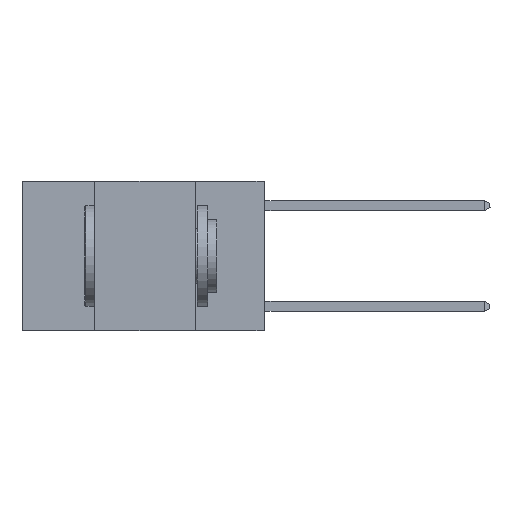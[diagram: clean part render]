
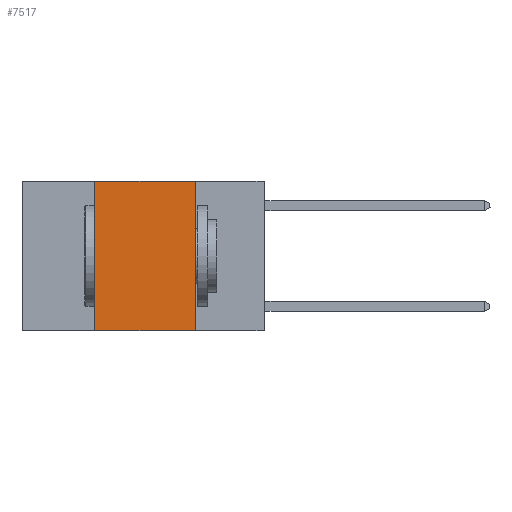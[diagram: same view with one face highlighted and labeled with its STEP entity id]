
A CAD part, left-side view. The second image highlights one B-rep face of the part: STEP entity #7517.
In plain terms, the highlighted planar face has unit normal (-1, 0, 0).
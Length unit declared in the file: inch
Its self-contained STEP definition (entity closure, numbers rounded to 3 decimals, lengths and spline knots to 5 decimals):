
#131 = ORIENTED_EDGE ( 'NONE', *, *, #8735, .F. ) ;
#279 = VECTOR ( 'NONE', #12831, 39.37008 ) ;
#870 = LINE ( 'NONE', #11042, #279 ) ;
#954 = VECTOR ( 'NONE', #21977, 39.37008 ) ;
#1001 = LINE ( 'NONE', #16248, #19426 ) ;
#1195 = DIRECTION ( 'NONE',  ( 0., 0., 1. ) ) ;
#1799 = FACE_OUTER_BOUND ( 'NONE', #18505, .T. ) ;
#2193 = DIRECTION ( 'NONE',  ( 0., 0., -1. ) ) ;
#2596 = CARTESIAN_POINT ( 'NONE',  ( 0., 0.17, 0. ) ) ;
#3584 = VERTEX_POINT ( 'NONE', #2596 ) ;
#5113 = EDGE_CURVE ( 'NONE', #10311, #12222, #20253, .T. ) ;
#5422 = EDGE_CURVE ( 'NONE', #12222, #3584, #1001, .T. ) ;
#6309 = EDGE_CURVE ( 'NONE', #10311, #13039, #10556, .T. ) ;
#7423 = DIRECTION ( 'NONE',  ( 0., -1., 0. ) ) ;
#7517 = ADVANCED_FACE ( 'NONE', ( #1799 ), #11163, .F. ) ;
#7858 = CARTESIAN_POINT ( 'NONE',  ( 0., 0.6, -0.37 ) ) ;
#8735 = EDGE_CURVE ( 'NONE', #3584, #13039, #870, .T. ) ;
#10311 = VERTEX_POINT ( 'NONE', #11741 ) ;
#10556 = LINE ( 'NONE', #7858, #954 ) ;
#11042 = CARTESIAN_POINT ( 'NONE',  ( 0., 0.17, 0. ) ) ;
#11163 = PLANE ( 'NONE',  #20207 ) ;
#11741 = CARTESIAN_POINT ( 'NONE',  ( 0., 0.42, -0.37 ) ) ;
#12222 = VERTEX_POINT ( 'NONE', #16903 ) ;
#12831 = DIRECTION ( 'NONE',  ( 0., 0., -1. ) ) ;
#12948 = DIRECTION ( 'NONE',  ( 1., 0., 0. ) ) ;
#13039 = VERTEX_POINT ( 'NONE', #13745 ) ;
#13625 = ORIENTED_EDGE ( 'NONE', *, *, #6309, .T. ) ;
#13745 = CARTESIAN_POINT ( 'NONE',  ( 0., 0.17, -0.37 ) ) ;
#14066 = ORIENTED_EDGE ( 'NONE', *, *, #5113, .F. ) ;
#15585 = VECTOR ( 'NONE', #1195, 39.37008 ) ;
#16248 = CARTESIAN_POINT ( 'NONE',  ( 0., 0.6, 0. ) ) ;
#16385 = ORIENTED_EDGE ( 'NONE', *, *, #5422, .F. ) ;
#16903 = CARTESIAN_POINT ( 'NONE',  ( 0., 0.42, 0. ) ) ;
#17201 = CARTESIAN_POINT ( 'NONE',  ( 0., 0.42, 0. ) ) ;
#18505 = EDGE_LOOP ( 'NONE', ( #131, #16385, #14066, #13625 ) ) ;
#19426 = VECTOR ( 'NONE', #7423, 39.37008 ) ;
#20207 = AXIS2_PLACEMENT_3D ( 'NONE', #21700, #12948, #2193 ) ;
#20253 = LINE ( 'NONE', #17201, #15585 ) ;
#21700 = CARTESIAN_POINT ( 'NONE',  ( 0., 0.6, 0. ) ) ;
#21977 = DIRECTION ( 'NONE',  ( 0., -1., 0. ) ) ;
